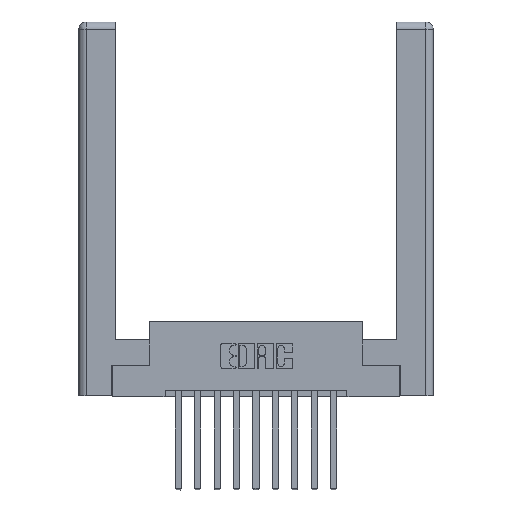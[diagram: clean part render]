
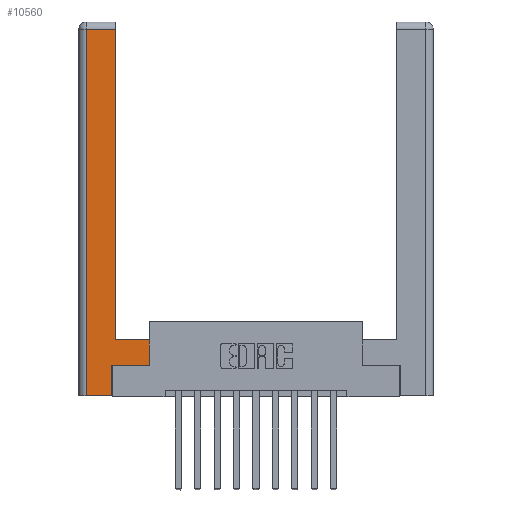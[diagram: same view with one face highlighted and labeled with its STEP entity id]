
A CAD part, top view. The second image highlights one B-rep face of the part: STEP entity #10560.
In plain terms, the highlighted planar face has unit normal (0, 0, 1).
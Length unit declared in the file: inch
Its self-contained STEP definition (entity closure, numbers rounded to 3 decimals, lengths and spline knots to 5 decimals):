
#78 = DIRECTION ( 'NONE',  ( 0., -1., 0. ) ) ;
#151 = LINE ( 'NONE', #13177, #812 ) ;
#199 = CARTESIAN_POINT ( 'NONE',  ( 0.265, 0.245, 0. ) ) ;
#341 = CARTESIAN_POINT ( 'NONE',  ( 0.565, 0.45, 0. ) ) ;
#591 = ORIENTED_EDGE ( 'NONE', *, *, #7935, .T. ) ;
#812 = VECTOR ( 'NONE', #7936, 39.37008 ) ;
#825 = CARTESIAN_POINT ( 'NONE',  ( 0.295, 0.45, 0. ) ) ;
#891 = CARTESIAN_POINT ( 'NONE',  ( 0.0615, 2.94, 0. ) ) ;
#1133 = VERTEX_POINT ( 'NONE', #825 ) ;
#1135 = VECTOR ( 'NONE', #6297, 39.37008 ) ;
#1477 = ORIENTED_EDGE ( 'NONE', *, *, #6520, .T. ) ;
#1576 = LINE ( 'NONE', #5132, #3240 ) ;
#1580 = DIRECTION ( 'NONE',  ( 0., 1., 0. ) ) ;
#2144 = ORIENTED_EDGE ( 'NONE', *, *, #11978, .T. ) ;
#2992 = EDGE_CURVE ( 'NONE', #9554, #13680, #151, .T. ) ;
#3240 = VECTOR ( 'NONE', #78, 39.37008 ) ;
#3697 = EDGE_CURVE ( 'NONE', #7230, #10993, #6898, .T. ) ;
#3838 = LINE ( 'NONE', #8308, #6461 ) ;
#4470 = ORIENTED_EDGE ( 'NONE', *, *, #3697, .T. ) ;
#4614 = ORIENTED_EDGE ( 'NONE', *, *, #10569, .T. ) ;
#5132 = CARTESIAN_POINT ( 'NONE',  ( 0.0615, 0., 0. ) ) ;
#5428 = ORIENTED_EDGE ( 'NONE', *, *, #9495, .T. ) ;
#5533 = VECTOR ( 'NONE', #7641, 39.37008 ) ;
#6141 = CARTESIAN_POINT ( 'NONE',  ( 0.0615, 0., 0. ) ) ;
#6297 = DIRECTION ( 'NONE',  ( 1., 0., 0. ) ) ;
#6389 = LINE ( 'NONE', #11747, #1135 ) ;
#6461 = VECTOR ( 'NONE', #9388, 39.37008 ) ;
#6520 = EDGE_CURVE ( 'NONE', #13680, #9496, #10612, .T. ) ;
#6652 = AXIS2_PLACEMENT_3D ( 'NONE', #7336, #8557, #9441 ) ;
#6742 = CARTESIAN_POINT ( 'NONE',  ( 0.265, 0.245, 0. ) ) ;
#6898 = LINE ( 'NONE', #891, #13545 ) ;
#7230 = VERTEX_POINT ( 'NONE', #10355 ) ;
#7255 = DIRECTION ( 'NONE',  ( -1., 0., 0. ) ) ;
#7336 = CARTESIAN_POINT ( 'NONE',  ( 0., 0., 0. ) ) ;
#7496 = ORIENTED_EDGE ( 'NONE', *, *, #12863, .T. ) ;
#7580 = DIRECTION ( 'NONE',  ( 0., 1., 0. ) ) ;
#7641 = DIRECTION ( 'NONE',  ( 0., 1., 0. ) ) ;
#7888 = CARTESIAN_POINT ( 'NONE',  ( 0.0615, 2.94, 0. ) ) ;
#7935 = EDGE_CURVE ( 'NONE', #9314, #10937, #6389, .T. ) ;
#7936 = DIRECTION ( 'NONE',  ( 1., 0., 0. ) ) ;
#8136 = VECTOR ( 'NONE', #1580, 39.37008 ) ;
#8224 = LINE ( 'NONE', #10853, #5533 ) ;
#8308 = CARTESIAN_POINT ( 'NONE',  ( 0.295, 0.45, 0. ) ) ;
#8557 = DIRECTION ( 'NONE',  ( 0., 0., -1. ) ) ;
#8586 = EDGE_LOOP ( 'NONE', ( #5428, #4470, #4614, #591, #7496, #10974, #1477, #2144 ) ) ;
#8622 = CARTESIAN_POINT ( 'NONE',  ( 0.565, 0.45, 0. ) ) ;
#8629 = VECTOR ( 'NONE', #7580, 39.37008 ) ;
#8890 = CARTESIAN_POINT ( 'NONE',  ( 0.265, 0., 0. ) ) ;
#9030 = FACE_OUTER_BOUND ( 'NONE', #8586, .T. ) ;
#9314 = VERTEX_POINT ( 'NONE', #6141 ) ;
#9388 = DIRECTION ( 'NONE',  ( -1., 0., 0. ) ) ;
#9441 = DIRECTION ( 'NONE',  ( -1., 0., 0. ) ) ;
#9495 = EDGE_CURVE ( 'NONE', #1133, #7230, #8224, .T. ) ;
#9496 = VERTEX_POINT ( 'NONE', #341 ) ;
#9554 = VERTEX_POINT ( 'NONE', #199 ) ;
#10355 = CARTESIAN_POINT ( 'NONE',  ( 0.295, 2.94, 0. ) ) ;
#10560 = ADVANCED_FACE ( 'NONE', ( #9030 ), #11502, .F. ) ;
#10569 = EDGE_CURVE ( 'NONE', #10993, #9314, #1576, .T. ) ;
#10612 = LINE ( 'NONE', #8622, #8629 ) ;
#10853 = CARTESIAN_POINT ( 'NONE',  ( 0.295, 3., 0. ) ) ;
#10937 = VERTEX_POINT ( 'NONE', #8890 ) ;
#10974 = ORIENTED_EDGE ( 'NONE', *, *, #2992, .T. ) ;
#10993 = VERTEX_POINT ( 'NONE', #7888 ) ;
#11125 = LINE ( 'NONE', #6742, #8136 ) ;
#11274 = CARTESIAN_POINT ( 'NONE',  ( 0.565, 0.245, 0. ) ) ;
#11502 = PLANE ( 'NONE',  #6652 ) ;
#11747 = CARTESIAN_POINT ( 'NONE',  ( 0.265, 0., 0. ) ) ;
#11978 = EDGE_CURVE ( 'NONE', #9496, #1133, #3838, .T. ) ;
#12863 = EDGE_CURVE ( 'NONE', #10937, #9554, #11125, .T. ) ;
#13177 = CARTESIAN_POINT ( 'NONE',  ( 0.565, 0.245, 0. ) ) ;
#13545 = VECTOR ( 'NONE', #7255, 39.37008 ) ;
#13680 = VERTEX_POINT ( 'NONE', #11274 ) ;
